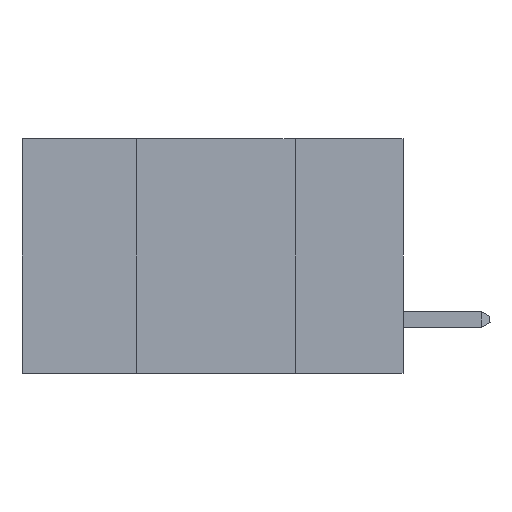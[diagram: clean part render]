
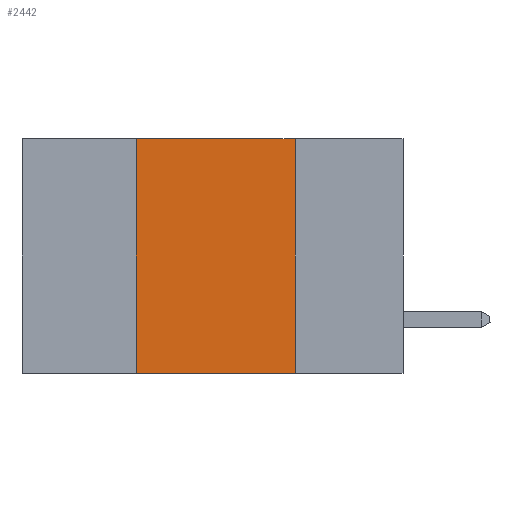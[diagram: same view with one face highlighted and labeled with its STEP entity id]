
A CAD part, left-side view. The second image highlights one B-rep face of the part: STEP entity #2442.
In plain terms, the highlighted planar face has unit normal (-1, 0, 0).
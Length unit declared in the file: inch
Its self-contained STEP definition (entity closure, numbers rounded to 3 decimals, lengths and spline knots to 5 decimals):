
#164 = CARTESIAN_POINT ( 'NONE',  ( 0., 0.17, 0. ) ) ;
#431 = CARTESIAN_POINT ( 'NONE',  ( 0., 0.6, 0. ) ) ;
#1990 = DIRECTION ( 'NONE',  ( 0., -1., 0. ) ) ;
#2442 = ADVANCED_FACE ( 'NONE', ( #13148 ), #12785, .F. ) ;
#2749 = VECTOR ( 'NONE', #12225, 39.37008 ) ;
#3464 = CARTESIAN_POINT ( 'NONE',  ( 0., 0.42, 0. ) ) ;
#3597 = CARTESIAN_POINT ( 'NONE',  ( 0., 0.17, -0.37 ) ) ;
#4175 = VERTEX_POINT ( 'NONE', #164 ) ;
#4475 = AXIS2_PLACEMENT_3D ( 'NONE', #15553, #12795, #16419 ) ;
#4838 = VERTEX_POINT ( 'NONE', #13316 ) ;
#5343 = EDGE_CURVE ( 'NONE', #4175, #5901, #6704, .T. ) ;
#5901 = VERTEX_POINT ( 'NONE', #3597 ) ;
#6551 = EDGE_CURVE ( 'NONE', #4838, #5901, #6583, .T. ) ;
#6562 = VERTEX_POINT ( 'NONE', #3464 ) ;
#6583 = LINE ( 'NONE', #13745, #2749 ) ;
#6704 = LINE ( 'NONE', #15281, #18222 ) ;
#8079 = EDGE_CURVE ( 'NONE', #6562, #4175, #15811, .T. ) ;
#9195 = ORIENTED_EDGE ( 'NONE', *, *, #8079, .F. ) ;
#9795 = ORIENTED_EDGE ( 'NONE', *, *, #6551, .T. ) ;
#10070 = LINE ( 'NONE', #17700, #16369 ) ;
#11243 = EDGE_CURVE ( 'NONE', #4838, #6562, #10070, .T. ) ;
#11608 = ORIENTED_EDGE ( 'NONE', *, *, #5343, .F. ) ;
#12225 = DIRECTION ( 'NONE',  ( 0., -1., 0. ) ) ;
#12505 = DIRECTION ( 'NONE',  ( 0., 0., -1. ) ) ;
#12785 = PLANE ( 'NONE',  #4475 ) ;
#12795 = DIRECTION ( 'NONE',  ( 1., 0., 0. ) ) ;
#13148 = FACE_OUTER_BOUND ( 'NONE', #17923, .T. ) ;
#13316 = CARTESIAN_POINT ( 'NONE',  ( 0., 0.42, -0.37 ) ) ;
#13745 = CARTESIAN_POINT ( 'NONE',  ( 0., 0.6, -0.37 ) ) ;
#15281 = CARTESIAN_POINT ( 'NONE',  ( 0., 0.17, 0. ) ) ;
#15553 = CARTESIAN_POINT ( 'NONE',  ( 0., 0.6, 0. ) ) ;
#15811 = LINE ( 'NONE', #431, #16018 ) ;
#16018 = VECTOR ( 'NONE', #1990, 39.37008 ) ;
#16369 = VECTOR ( 'NONE', #18536, 39.37008 ) ;
#16419 = DIRECTION ( 'NONE',  ( 0., 0., -1. ) ) ;
#17700 = CARTESIAN_POINT ( 'NONE',  ( 0., 0.42, 0. ) ) ;
#17923 = EDGE_LOOP ( 'NONE', ( #11608, #9195, #18249, #9795 ) ) ;
#18222 = VECTOR ( 'NONE', #12505, 39.37008 ) ;
#18249 = ORIENTED_EDGE ( 'NONE', *, *, #11243, .F. ) ;
#18536 = DIRECTION ( 'NONE',  ( 0., 0., 1. ) ) ;
